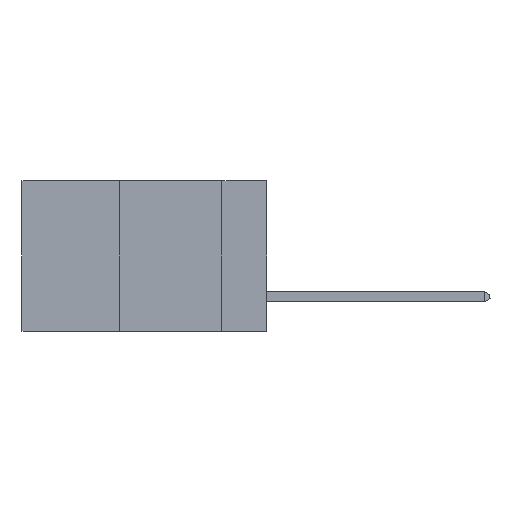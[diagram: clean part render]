
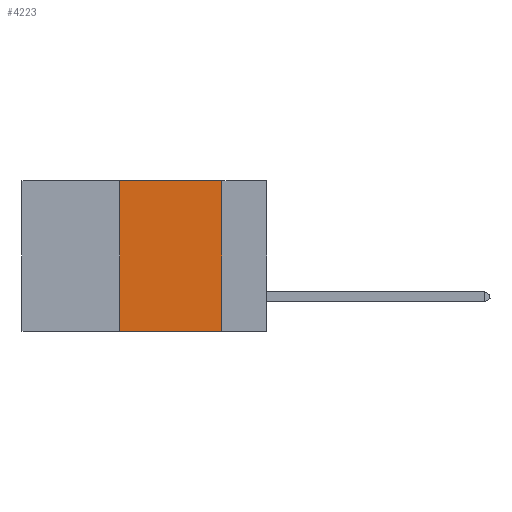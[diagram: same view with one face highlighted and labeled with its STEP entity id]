
A CAD part, left-side view. The second image highlights one B-rep face of the part: STEP entity #4223.
In plain terms, the highlighted planar face has unit normal (-1, 0, 0).
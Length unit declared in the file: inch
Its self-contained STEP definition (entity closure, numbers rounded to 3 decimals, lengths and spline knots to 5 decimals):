
#426 = VERTEX_POINT ( 'NONE', #4150 ) ;
#593 = PLANE ( 'NONE',  #10489 ) ;
#675 = FACE_OUTER_BOUND ( 'NONE', #11195, .T. ) ;
#746 = DIRECTION ( 'NONE',  ( 0., -1., 0. ) ) ;
#754 = ORIENTED_EDGE ( 'NONE', *, *, #6784, .F. ) ;
#1161 = CARTESIAN_POINT ( 'NONE',  ( 0., 0.36, -0.37 ) ) ;
#1740 = VECTOR ( 'NONE', #10628, 39.37008 ) ;
#1957 = VECTOR ( 'NONE', #3973, 39.37008 ) ;
#2846 = EDGE_CURVE ( 'NONE', #6679, #426, #8426, .T. ) ;
#3675 = DIRECTION ( 'NONE',  ( 0., 0., 1. ) ) ;
#3973 = DIRECTION ( 'NONE',  ( 0., -1., 0. ) ) ;
#4018 = DIRECTION ( 'NONE',  ( 1., 0., 0. ) ) ;
#4150 = CARTESIAN_POINT ( 'NONE',  ( 0., 0.11, -0.37 ) ) ;
#4223 = ADVANCED_FACE ( 'NONE', ( #675 ), #593, .F. ) ;
#4450 = EDGE_CURVE ( 'NONE', #6679, #7684, #10438, .T. ) ;
#5035 = LINE ( 'NONE', #8407, #1957 ) ;
#5379 = CARTESIAN_POINT ( 'NONE',  ( 0., 0.11, 0. ) ) ;
#5461 = ORIENTED_EDGE ( 'NONE', *, *, #2846, .T. ) ;
#6054 = EDGE_CURVE ( 'NONE', #6678, #426, #9723, .T. ) ;
#6149 = CARTESIAN_POINT ( 'NONE',  ( 0., 0.6, 0. ) ) ;
#6330 = CARTESIAN_POINT ( 'NONE',  ( 0., 0.11, 0. ) ) ;
#6358 = VECTOR ( 'NONE', #746, 39.37008 ) ;
#6365 = CARTESIAN_POINT ( 'NONE',  ( 0., 0.36, 0. ) ) ;
#6678 = VERTEX_POINT ( 'NONE', #6330 ) ;
#6679 = VERTEX_POINT ( 'NONE', #1161 ) ;
#6784 = EDGE_CURVE ( 'NONE', #7684, #6678, #5035, .T. ) ;
#7207 = CARTESIAN_POINT ( 'NONE',  ( 0., 0.36, 0. ) ) ;
#7684 = VERTEX_POINT ( 'NONE', #6365 ) ;
#7706 = DIRECTION ( 'NONE',  ( 0., 0., -1. ) ) ;
#8126 = VECTOR ( 'NONE', #3675, 39.37008 ) ;
#8308 = ORIENTED_EDGE ( 'NONE', *, *, #4450, .F. ) ;
#8407 = CARTESIAN_POINT ( 'NONE',  ( 0., 0.6, 0. ) ) ;
#8426 = LINE ( 'NONE', #8684, #6358 ) ;
#8684 = CARTESIAN_POINT ( 'NONE',  ( 0., 0.6, -0.37 ) ) ;
#9141 = ORIENTED_EDGE ( 'NONE', *, *, #6054, .F. ) ;
#9723 = LINE ( 'NONE', #5379, #1740 ) ;
#10438 = LINE ( 'NONE', #7207, #8126 ) ;
#10489 = AXIS2_PLACEMENT_3D ( 'NONE', #6149, #4018, #7706 ) ;
#10628 = DIRECTION ( 'NONE',  ( 0., 0., -1. ) ) ;
#11195 = EDGE_LOOP ( 'NONE', ( #9141, #754, #8308, #5461 ) ) ;
